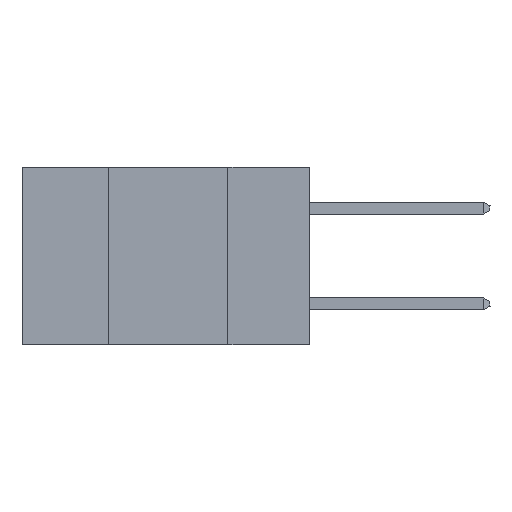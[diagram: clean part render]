
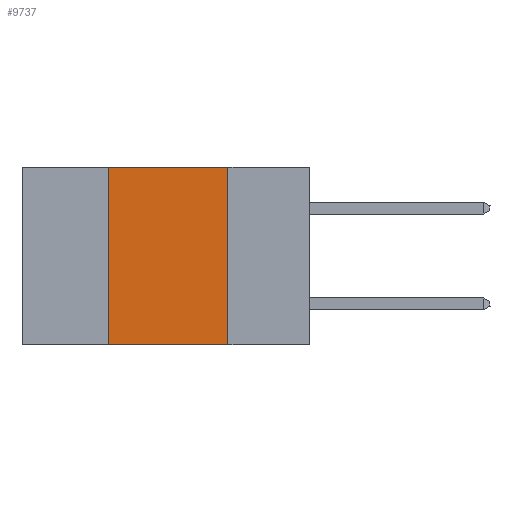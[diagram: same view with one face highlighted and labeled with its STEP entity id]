
A CAD part, left-side view. The second image highlights one B-rep face of the part: STEP entity #9737.
In plain terms, the highlighted planar face has unit normal (-1, 0, 0).
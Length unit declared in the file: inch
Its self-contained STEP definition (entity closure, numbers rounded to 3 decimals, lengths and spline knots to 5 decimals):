
#178 = ORIENTED_EDGE ( 'NONE', *, *, #6263, .F. ) ;
#348 = DIRECTION ( 'NONE',  ( 0., -1., 0. ) ) ;
#492 = LINE ( 'NONE', #6953, #5466 ) ;
#758 = DIRECTION ( 'NONE',  ( 0., 0., 1. ) ) ;
#1156 = CARTESIAN_POINT ( 'NONE',  ( 0., 0.42, -0.37 ) ) ;
#1715 = CARTESIAN_POINT ( 'NONE',  ( 0., 0.42, 0. ) ) ;
#2414 = CARTESIAN_POINT ( 'NONE',  ( 0., 0.6, 0. ) ) ;
#2725 = ORIENTED_EDGE ( 'NONE', *, *, #3114, .T. ) ;
#2789 = CARTESIAN_POINT ( 'NONE',  ( 0., 0.42, 0. ) ) ;
#3059 = EDGE_CURVE ( 'NONE', #12830, #5021, #8370, .T. ) ;
#3114 = EDGE_CURVE ( 'NONE', #5546, #7441, #492, .T. ) ;
#3255 = VECTOR ( 'NONE', #11444, 39.37008 ) ;
#3451 = LINE ( 'NONE', #2789, #10977 ) ;
#3995 = DIRECTION ( 'NONE',  ( 0., -1., 0. ) ) ;
#5021 = VERTEX_POINT ( 'NONE', #11038 ) ;
#5352 = EDGE_LOOP ( 'NONE', ( #178, #7660, #7897, #2725 ) ) ;
#5466 = VECTOR ( 'NONE', #3995, 39.37008 ) ;
#5546 = VERTEX_POINT ( 'NONE', #1156 ) ;
#5686 = CARTESIAN_POINT ( 'NONE',  ( 0., 0.17, 0. ) ) ;
#6263 = EDGE_CURVE ( 'NONE', #5021, #7441, #11399, .T. ) ;
#6778 = CARTESIAN_POINT ( 'NONE',  ( 0., 0.6, 0. ) ) ;
#6811 = VECTOR ( 'NONE', #348, 39.37008 ) ;
#6953 = CARTESIAN_POINT ( 'NONE',  ( 0., 0.6, -0.37 ) ) ;
#7441 = VERTEX_POINT ( 'NONE', #8508 ) ;
#7660 = ORIENTED_EDGE ( 'NONE', *, *, #3059, .F. ) ;
#7897 = ORIENTED_EDGE ( 'NONE', *, *, #9367, .F. ) ;
#8370 = LINE ( 'NONE', #2414, #6811 ) ;
#8508 = CARTESIAN_POINT ( 'NONE',  ( 0., 0.17, -0.37 ) ) ;
#8688 = DIRECTION ( 'NONE',  ( 0., 0., -1. ) ) ;
#9367 = EDGE_CURVE ( 'NONE', #5546, #12830, #3451, .T. ) ;
#9419 = FACE_OUTER_BOUND ( 'NONE', #5352, .T. ) ;
#9737 = ADVANCED_FACE ( 'NONE', ( #9419 ), #10667, .F. ) ;
#10667 = PLANE ( 'NONE',  #12690 ) ;
#10800 = DIRECTION ( 'NONE',  ( 1., 0., 0. ) ) ;
#10977 = VECTOR ( 'NONE', #758, 39.37008 ) ;
#11038 = CARTESIAN_POINT ( 'NONE',  ( 0., 0.17, 0. ) ) ;
#11399 = LINE ( 'NONE', #5686, #3255 ) ;
#11444 = DIRECTION ( 'NONE',  ( 0., 0., -1. ) ) ;
#12690 = AXIS2_PLACEMENT_3D ( 'NONE', #6778, #10800, #8688 ) ;
#12830 = VERTEX_POINT ( 'NONE', #1715 ) ;
